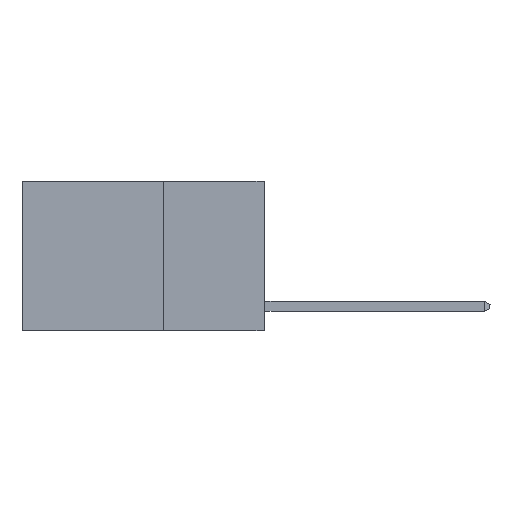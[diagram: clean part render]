
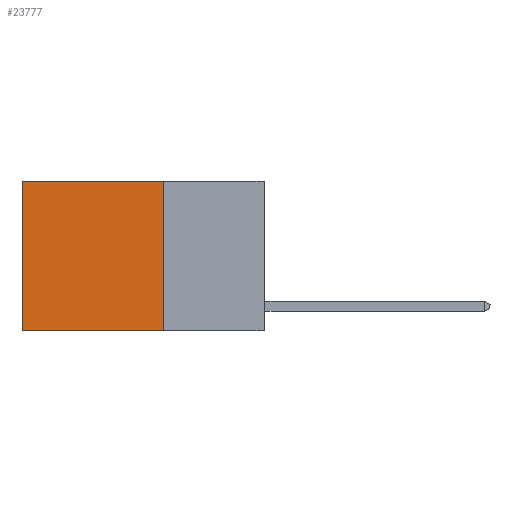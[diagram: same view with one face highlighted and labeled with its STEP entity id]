
A CAD part, left-side view. The second image highlights one B-rep face of the part: STEP entity #23777.
In plain terms, the highlighted planar face has unit normal (-1, 0, 0).
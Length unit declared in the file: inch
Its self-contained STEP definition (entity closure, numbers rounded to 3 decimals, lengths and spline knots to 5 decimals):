
#424 = EDGE_CURVE ( 'NONE', #13247, #9692, #10317, .T. ) ;
#1761 = CARTESIAN_POINT ( 'NONE',  ( 0.2625, 0.25, 0. ) ) ;
#1864 = LINE ( 'NONE', #7757, #22318 ) ;
#1951 = FACE_OUTER_BOUND ( 'NONE', #2202, .T. ) ;
#2202 = EDGE_LOOP ( 'NONE', ( #12407, #16687, #21283, #5826 ) ) ;
#3494 = DIRECTION ( 'NONE',  ( 0., 0., -1. ) ) ;
#3613 = DIRECTION ( 'NONE',  ( 0., 1., 0. ) ) ;
#3896 = CARTESIAN_POINT ( 'NONE',  ( 0.2625, 0.25, 0. ) ) ;
#4433 = EDGE_CURVE ( 'NONE', #20150, #13247, #1864, .T. ) ;
#5187 = DIRECTION ( 'NONE',  ( 1., 0., 0. ) ) ;
#5731 = CARTESIAN_POINT ( 'NONE',  ( 0.2625, 0.25, -0.37 ) ) ;
#5826 = ORIENTED_EDGE ( 'NONE', *, *, #11666, .T. ) ;
#7143 = VECTOR ( 'NONE', #14568, 39.37008 ) ;
#7757 = CARTESIAN_POINT ( 'NONE',  ( 0.2625, 0.25, 0. ) ) ;
#8996 = PLANE ( 'NONE',  #11882 ) ;
#9559 = DIRECTION ( 'NONE',  ( 0., 0., -1. ) ) ;
#9692 = VERTEX_POINT ( 'NONE', #14997 ) ;
#10317 = LINE ( 'NONE', #21799, #7143 ) ;
#10844 = DIRECTION ( 'NONE',  ( 0., 0., -1. ) ) ;
#11666 = EDGE_CURVE ( 'NONE', #20150, #16577, #17422, .T. ) ;
#11882 = AXIS2_PLACEMENT_3D ( 'NONE', #20079, #5187, #10844 ) ;
#12407 = ORIENTED_EDGE ( 'NONE', *, *, #23073, .T. ) ;
#12497 = VECTOR ( 'NONE', #3613, 39.37008 ) ;
#13247 = VERTEX_POINT ( 'NONE', #5731 ) ;
#14568 = DIRECTION ( 'NONE',  ( 0., 1., 0. ) ) ;
#14997 = CARTESIAN_POINT ( 'NONE',  ( 0.2625, 0.6, -0.37 ) ) ;
#16577 = VERTEX_POINT ( 'NONE', #20199 ) ;
#16687 = ORIENTED_EDGE ( 'NONE', *, *, #424, .F. ) ;
#17422 = LINE ( 'NONE', #1761, #12497 ) ;
#18018 = CARTESIAN_POINT ( 'NONE',  ( 0.2625, 0.6, 0. ) ) ;
#20079 = CARTESIAN_POINT ( 'NONE',  ( 0.2625, 0.25, 0. ) ) ;
#20150 = VERTEX_POINT ( 'NONE', #3896 ) ;
#20199 = CARTESIAN_POINT ( 'NONE',  ( 0.2625, 0.6, 0. ) ) ;
#21283 = ORIENTED_EDGE ( 'NONE', *, *, #4433, .F. ) ;
#21799 = CARTESIAN_POINT ( 'NONE',  ( 0.2625, 0.25, -0.37 ) ) ;
#22318 = VECTOR ( 'NONE', #9559, 39.37008 ) ;
#22737 = LINE ( 'NONE', #18018, #23315 ) ;
#23073 = EDGE_CURVE ( 'NONE', #16577, #9692, #22737, .T. ) ;
#23315 = VECTOR ( 'NONE', #3494, 39.37008 ) ;
#23777 = ADVANCED_FACE ( 'NONE', ( #1951 ), #8996, .F. ) ;
